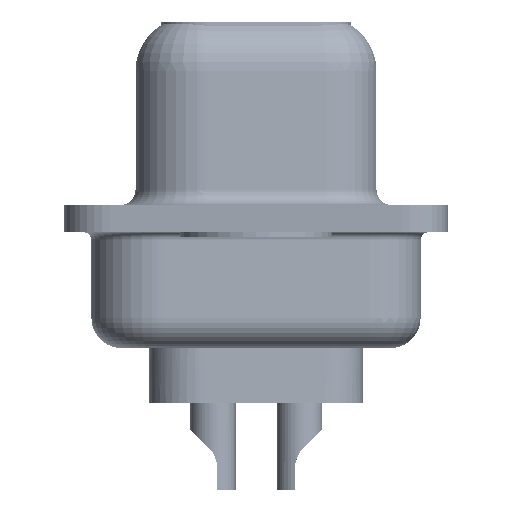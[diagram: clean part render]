
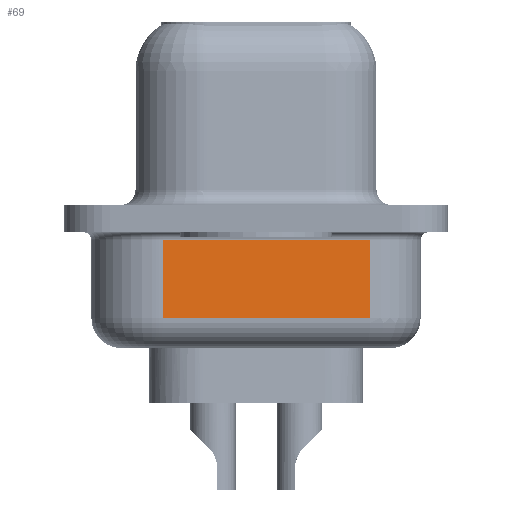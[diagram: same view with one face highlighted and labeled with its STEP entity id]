
A CAD part, left-side view. The second image highlights one B-rep face of the part: STEP entity #69.
In plain terms, the highlighted planar face has unit normal (-0.985, -0.174, 0).
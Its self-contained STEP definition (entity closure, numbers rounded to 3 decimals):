
#69 = ADVANCED_FACE ( 'NONE', ( #4125 ), #11674, .F. ) ;
#913 = ORIENTED_EDGE ( 'NONE', *, *, #2291, .T. ) ;
#954 = AXIS2_PLACEMENT_3D ( 'NONE', #24356, #13806, #958 ) ;
#958 = DIRECTION ( 'NONE',  ( -0.174, 0.985, 0. ) ) ;
#1598 = ORIENTED_EDGE ( 'NONE', *, *, #27085, .T. ) ;
#1696 = CARTESIAN_POINT ( 'NONE',  ( 2.88, 3.053, -3.25 ) ) ;
#2291 = EDGE_CURVE ( 'NONE', #21104, #17752, #13688, .T. ) ;
#2505 = CARTESIAN_POINT ( 'NONE',  ( 2.88, 3.053, -4.25 ) ) ;
#2751 = LINE ( 'NONE', #4402, #6398 ) ;
#4002 = LINE ( 'NONE', #7630, #15379 ) ;
#4125 = FACE_OUTER_BOUND ( 'NONE', #6271, .T. ) ;
#4402 = CARTESIAN_POINT ( 'NONE',  ( 4.079, -3.747, -4.25 ) ) ;
#6271 = EDGE_LOOP ( 'NONE', ( #11898, #913, #10215, #1598 ) ) ;
#6376 = VECTOR ( 'NONE', #25891, 1000. ) ;
#6398 = VECTOR ( 'NONE', #19329, 1000. ) ;
#7630 = CARTESIAN_POINT ( 'NONE',  ( 2.88, 3.053, -0.7 ) ) ;
#10215 = ORIENTED_EDGE ( 'NONE', *, *, #10381, .T. ) ;
#10381 = EDGE_CURVE ( 'NONE', #17752, #15804, #2751, .T. ) ;
#10499 = CARTESIAN_POINT ( 'NONE',  ( 2.88, 3.053, -3.25 ) ) ;
#10751 = CARTESIAN_POINT ( 'NONE',  ( 2.88, 3.053, -0.7 ) ) ;
#10933 = EDGE_CURVE ( 'NONE', #21104, #21475, #17725, .T. ) ;
#11674 = PLANE ( 'NONE',  #954 ) ;
#11898 = ORIENTED_EDGE ( 'NONE', *, *, #10933, .F. ) ;
#12368 = VECTOR ( 'NONE', #21786, 1000. ) ;
#13688 = LINE ( 'NONE', #1696, #12368 ) ;
#13806 = DIRECTION ( 'NONE',  ( 0.985, 0.174, 0. ) ) ;
#15299 = CARTESIAN_POINT ( 'NONE',  ( 4.079, -3.747, -0.7 ) ) ;
#15379 = VECTOR ( 'NONE', #26768, 1000. ) ;
#15804 = VERTEX_POINT ( 'NONE', #15299 ) ;
#17725 = LINE ( 'NONE', #2505, #6376 ) ;
#17752 = VERTEX_POINT ( 'NONE', #20908 ) ;
#19329 = DIRECTION ( 'NONE',  ( 0., 0., 1. ) ) ;
#20908 = CARTESIAN_POINT ( 'NONE',  ( 4.079, -3.747, -3.25 ) ) ;
#21104 = VERTEX_POINT ( 'NONE', #10499 ) ;
#21475 = VERTEX_POINT ( 'NONE', #10751 ) ;
#21786 = DIRECTION ( 'NONE',  ( 0.174, -0.985, 0. ) ) ;
#24356 = CARTESIAN_POINT ( 'NONE',  ( 2.88, 3.053, -4.25 ) ) ;
#25891 = DIRECTION ( 'NONE',  ( 0., 0., 1. ) ) ;
#26768 = DIRECTION ( 'NONE',  ( -0.174, 0.985, 0. ) ) ;
#27085 = EDGE_CURVE ( 'NONE', #15804, #21475, #4002, .T. ) ;
